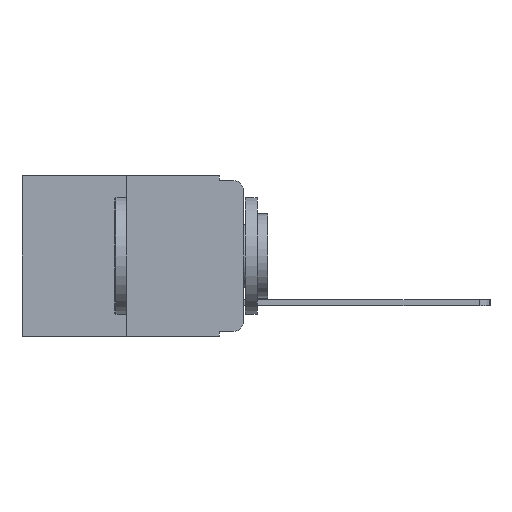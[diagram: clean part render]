
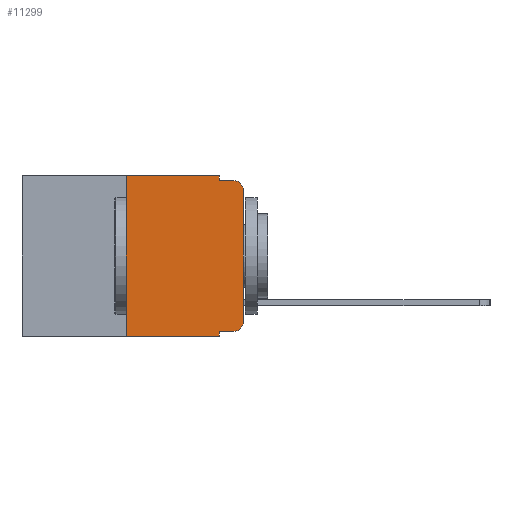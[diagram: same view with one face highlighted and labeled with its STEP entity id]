
A CAD part, left-side view. The second image highlights one B-rep face of the part: STEP entity #11299.
In plain terms, the highlighted planar face has unit normal (-1, 0, 0).
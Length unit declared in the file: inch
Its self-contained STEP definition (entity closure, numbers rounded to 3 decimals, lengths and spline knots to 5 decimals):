
#27 = VECTOR ( 'NONE', #5496, 39.37008 ) ;
#68 = EDGE_CURVE ( 'NONE', #9057, #7197, #4011, .T. ) ;
#141 = ORIENTED_EDGE ( 'NONE', *, *, #3468, .F. ) ;
#314 = ORIENTED_EDGE ( 'NONE', *, *, #5999, .F. ) ;
#321 = CARTESIAN_POINT ( 'NONE',  ( 0., 0., -0.03 ) ) ;
#393 = DIRECTION ( 'NONE',  ( 0., -1., 0. ) ) ;
#477 = ORIENTED_EDGE ( 'NONE', *, *, #6633, .T. ) ;
#569 = CARTESIAN_POINT ( 'NONE',  ( 0., 0.473, 0. ) ) ;
#659 = ORIENTED_EDGE ( 'NONE', *, *, #7279, .T. ) ;
#794 = EDGE_CURVE ( 'NONE', #2728, #9057, #11848, .T. ) ;
#805 = CARTESIAN_POINT ( 'NONE',  ( 0., 0.25, -0.343 ) ) ;
#816 = CARTESIAN_POINT ( 'NONE',  ( 0., 0.051, -0.01 ) ) ;
#1180 = CARTESIAN_POINT ( 'NONE',  ( 0., 0., 0. ) ) ;
#1480 = EDGE_CURVE ( 'NONE', #2728, #5151, #12275, .T. ) ;
#1636 = VECTOR ( 'NONE', #8922, 39.37008 ) ;
#1796 = ORIENTED_EDGE ( 'NONE', *, *, #68, .T. ) ;
#1834 = DIRECTION ( 'NONE',  ( -1., 0., 0. ) ) ;
#1974 = ORIENTED_EDGE ( 'NONE', *, *, #794, .T. ) ;
#2166 = EDGE_CURVE ( 'NONE', #7685, #2745, #2774, .T. ) ;
#2259 = DIRECTION ( 'NONE',  ( 0., 0., -1. ) ) ;
#2645 = DIRECTION ( 'NONE',  ( 1., 0., 0. ) ) ;
#2728 = VERTEX_POINT ( 'NONE', #10835 ) ;
#2745 = VERTEX_POINT ( 'NONE', #10770 ) ;
#2768 = CARTESIAN_POINT ( 'NONE',  ( 0., 0.02, -0.01 ) ) ;
#2774 = LINE ( 'NONE', #11644, #27 ) ;
#2887 = CARTESIAN_POINT ( 'NONE',  ( 0., 0.02, -0.313 ) ) ;
#2916 = CARTESIAN_POINT ( 'NONE',  ( 0., 0.051, -0.01 ) ) ;
#3468 = EDGE_CURVE ( 'NONE', #7884, #4881, #3931, .T. ) ;
#3626 = EDGE_CURVE ( 'NONE', #7685, #5151, #8361, .T. ) ;
#3663 = DIRECTION ( 'NONE',  ( -1., 0., 0. ) ) ;
#3803 = DIRECTION ( 'NONE',  ( 0., -1., 0. ) ) ;
#3931 = LINE ( 'NONE', #9899, #1636 ) ;
#4011 = CIRCLE ( 'NONE', #6254, 0.02 ) ;
#4422 = DIRECTION ( 'NONE',  ( 0., 0., -1. ) ) ;
#4458 = AXIS2_PLACEMENT_3D ( 'NONE', #569, #2645, #9213 ) ;
#4712 = LINE ( 'NONE', #8146, #11819 ) ;
#4881 = VERTEX_POINT ( 'NONE', #2916 ) ;
#4976 = CARTESIAN_POINT ( 'NONE',  ( 0., 0.02, -0.333 ) ) ;
#5151 = VERTEX_POINT ( 'NONE', #9926 ) ;
#5496 = DIRECTION ( 'NONE',  ( 0., 0., 1. ) ) ;
#5946 = VERTEX_POINT ( 'NONE', #2768 ) ;
#5999 = EDGE_CURVE ( 'NONE', #4881, #5946, #9531, .T. ) ;
#6254 = AXIS2_PLACEMENT_3D ( 'NONE', #2887, #3663, #2259 ) ;
#6468 = ORIENTED_EDGE ( 'NONE', *, *, #11208, .F. ) ;
#6503 = CARTESIAN_POINT ( 'NONE',  ( 0., 0.473, -0.343 ) ) ;
#6633 = EDGE_CURVE ( 'NONE', #7021, #5946, #10500, .T. ) ;
#6826 = ORIENTED_EDGE ( 'NONE', *, *, #1480, .F. ) ;
#6828 = CARTESIAN_POINT ( 'NONE',  ( 0., 0., -0.313 ) ) ;
#7021 = VERTEX_POINT ( 'NONE', #321 ) ;
#7063 = VECTOR ( 'NONE', #3803, 39.37008 ) ;
#7186 = VECTOR ( 'NONE', #9850, 39.37008 ) ;
#7197 = VERTEX_POINT ( 'NONE', #6828 ) ;
#7279 = EDGE_CURVE ( 'NONE', #7197, #7021, #10906, .T. ) ;
#7550 = CARTESIAN_POINT ( 'NONE',  ( 0., 0.02, -0.03 ) ) ;
#7685 = VERTEX_POINT ( 'NONE', #805 ) ;
#7711 = EDGE_LOOP ( 'NONE', ( #659, #477, #314, #141, #6468, #9395, #9741, #6826, #1974, #1796 ) ) ;
#7884 = VERTEX_POINT ( 'NONE', #11478 ) ;
#7893 = DIRECTION ( 'NONE',  ( 0., 0., 1. ) ) ;
#8146 = CARTESIAN_POINT ( 'NONE',  ( 0., 0.473, 0. ) ) ;
#8307 = PLANE ( 'NONE',  #4458 ) ;
#8361 = LINE ( 'NONE', #6503, #7186 ) ;
#8495 = DIRECTION ( 'NONE',  ( 0., 0., -1. ) ) ;
#8537 = FACE_OUTER_BOUND ( 'NONE', #7711, .T. ) ;
#8772 = VECTOR ( 'NONE', #7893, 39.37008 ) ;
#8922 = DIRECTION ( 'NONE',  ( 0., 0., -1. ) ) ;
#9057 = VERTEX_POINT ( 'NONE', #4976 ) ;
#9213 = DIRECTION ( 'NONE',  ( 0., 0., -1. ) ) ;
#9395 = ORIENTED_EDGE ( 'NONE', *, *, #2166, .F. ) ;
#9531 = LINE ( 'NONE', #816, #7063 ) ;
#9712 = VECTOR ( 'NONE', #11887, 39.37008 ) ;
#9741 = ORIENTED_EDGE ( 'NONE', *, *, #3626, .T. ) ;
#9843 = VECTOR ( 'NONE', #4422, 39.37008 ) ;
#9850 = DIRECTION ( 'NONE',  ( 0., -1., 0. ) ) ;
#9899 = CARTESIAN_POINT ( 'NONE',  ( 0., 0.051, 0. ) ) ;
#9926 = CARTESIAN_POINT ( 'NONE',  ( 0., 0.051, -0.343 ) ) ;
#10500 = CIRCLE ( 'NONE', #10722, 0.02 ) ;
#10586 = CARTESIAN_POINT ( 'NONE',  ( 0., 0.051, 0. ) ) ;
#10722 = AXIS2_PLACEMENT_3D ( 'NONE', #7550, #1834, #8495 ) ;
#10770 = CARTESIAN_POINT ( 'NONE',  ( 0., 0.25, 0. ) ) ;
#10835 = CARTESIAN_POINT ( 'NONE',  ( 0., 0.051, -0.333 ) ) ;
#10906 = LINE ( 'NONE', #1180, #8772 ) ;
#11208 = EDGE_CURVE ( 'NONE', #2745, #7884, #4712, .T. ) ;
#11299 = ADVANCED_FACE ( 'NONE', ( #8537 ), #8307, .F. ) ;
#11478 = CARTESIAN_POINT ( 'NONE',  ( 0., 0.051, 0. ) ) ;
#11644 = CARTESIAN_POINT ( 'NONE',  ( 0., 0.25, 0. ) ) ;
#11697 = CARTESIAN_POINT ( 'NONE',  ( 0., 0.051, -0.333 ) ) ;
#11819 = VECTOR ( 'NONE', #393, 39.37008 ) ;
#11848 = LINE ( 'NONE', #11697, #9712 ) ;
#11887 = DIRECTION ( 'NONE',  ( 0., -1., 0. ) ) ;
#12275 = LINE ( 'NONE', #10586, #9843 ) ;
